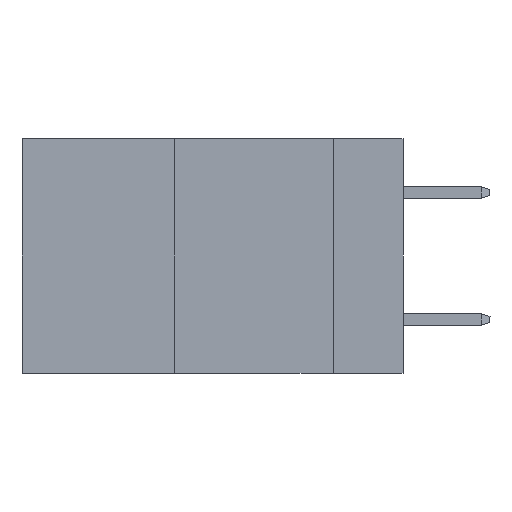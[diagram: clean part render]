
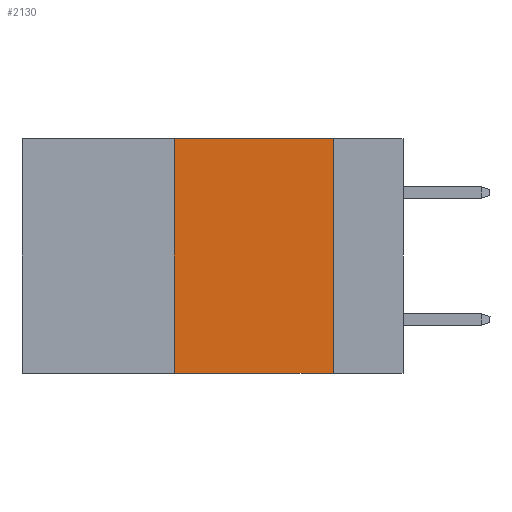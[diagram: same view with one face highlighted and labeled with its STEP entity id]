
A CAD part, left-side view. The second image highlights one B-rep face of the part: STEP entity #2130.
In plain terms, the highlighted planar face has unit normal (-1, 0, 0).
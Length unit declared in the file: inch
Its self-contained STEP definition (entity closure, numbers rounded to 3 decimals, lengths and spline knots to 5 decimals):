
#1 = EDGE_CURVE ( 'NONE', #8266, #1763, #7668, .T. ) ;
#264 = CARTESIAN_POINT ( 'NONE',  ( 0., 0.6, -0.37 ) ) ;
#807 = ORIENTED_EDGE ( 'NONE', *, *, #7936, .F. ) ;
#1184 = VERTEX_POINT ( 'NONE', #7631 ) ;
#1325 = VECTOR ( 'NONE', #5882, 39.37008 ) ;
#1336 = CARTESIAN_POINT ( 'NONE',  ( 0., 0.11, 0. ) ) ;
#1353 = CARTESIAN_POINT ( 'NONE',  ( 0., 0.36, 0. ) ) ;
#1690 = LINE ( 'NONE', #264, #1325 ) ;
#1763 = VERTEX_POINT ( 'NONE', #3728 ) ;
#2028 = DIRECTION ( 'NONE',  ( 0., 0., 1. ) ) ;
#2130 = ADVANCED_FACE ( 'NONE', ( #5999 ), #2562, .F. ) ;
#2239 = CARTESIAN_POINT ( 'NONE',  ( 0., 0.36, 0. ) ) ;
#2292 = CARTESIAN_POINT ( 'NONE',  ( 0., 0.6, 0. ) ) ;
#2562 = PLANE ( 'NONE',  #8961 ) ;
#2753 = DIRECTION ( 'NONE',  ( 0., 0., -1. ) ) ;
#3283 = ORIENTED_EDGE ( 'NONE', *, *, #8746, .F. ) ;
#3311 = ORIENTED_EDGE ( 'NONE', *, *, #8854, .T. ) ;
#3728 = CARTESIAN_POINT ( 'NONE',  ( 0., 0.11, -0.37 ) ) ;
#4150 = DIRECTION ( 'NONE',  ( 0., 0., -1. ) ) ;
#5882 = DIRECTION ( 'NONE',  ( 0., -1., 0. ) ) ;
#5999 = FACE_OUTER_BOUND ( 'NONE', #7716, .T. ) ;
#6039 = VECTOR ( 'NONE', #2028, 39.37008 ) ;
#6110 = LINE ( 'NONE', #2239, #6039 ) ;
#6251 = CARTESIAN_POINT ( 'NONE',  ( 0., 0.6, 0. ) ) ;
#6851 = VERTEX_POINT ( 'NONE', #1353 ) ;
#7057 = CARTESIAN_POINT ( 'NONE',  ( 0., 0.11, 0. ) ) ;
#7380 = VECTOR ( 'NONE', #7705, 39.37008 ) ;
#7617 = ORIENTED_EDGE ( 'NONE', *, *, #1, .F. ) ;
#7631 = CARTESIAN_POINT ( 'NONE',  ( 0., 0.36, -0.37 ) ) ;
#7668 = LINE ( 'NONE', #1336, #7740 ) ;
#7705 = DIRECTION ( 'NONE',  ( 0., -1., 0. ) ) ;
#7716 = EDGE_LOOP ( 'NONE', ( #7617, #3283, #807, #3311 ) ) ;
#7740 = VECTOR ( 'NONE', #4150, 39.37008 ) ;
#7936 = EDGE_CURVE ( 'NONE', #1184, #6851, #6110, .T. ) ;
#8266 = VERTEX_POINT ( 'NONE', #7057 ) ;
#8606 = LINE ( 'NONE', #2292, #7380 ) ;
#8746 = EDGE_CURVE ( 'NONE', #6851, #8266, #8606, .T. ) ;
#8854 = EDGE_CURVE ( 'NONE', #1184, #1763, #1690, .T. ) ;
#8961 = AXIS2_PLACEMENT_3D ( 'NONE', #6251, #9083, #2753 ) ;
#9083 = DIRECTION ( 'NONE',  ( 1., 0., 0. ) ) ;
